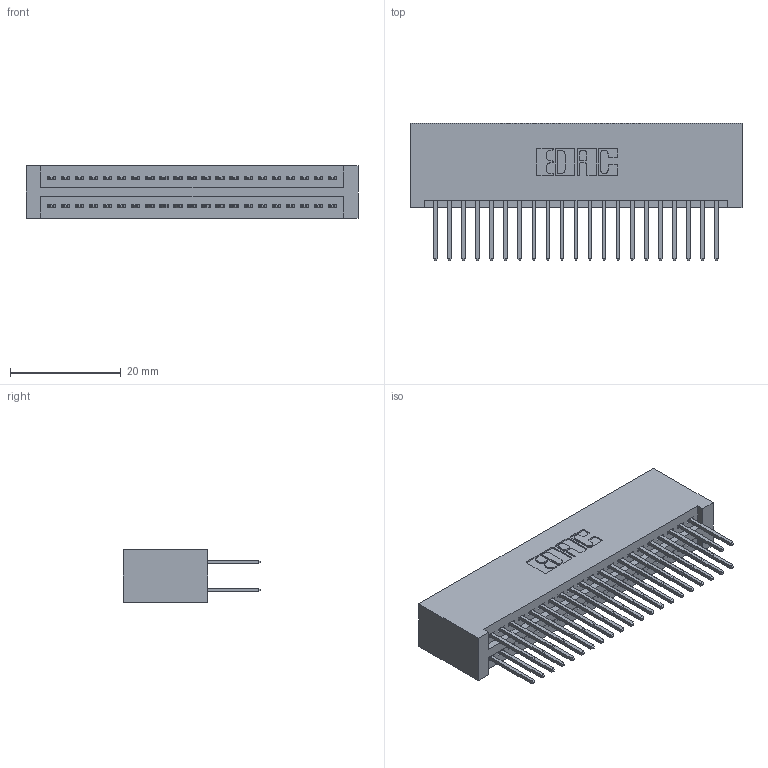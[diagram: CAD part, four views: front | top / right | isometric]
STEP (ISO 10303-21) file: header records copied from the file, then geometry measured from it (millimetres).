
FILE_DESCRIPTION (( 'STEP AP203' ), '1' );
FILE_NAME ('395-042-523-201.STEP', '2019-10-18T06:40:13', ( '' ), ( '' ), 'SwSTEP 2.0', 'SolidWorks 2016', '' );
FILE_SCHEMA (( 'CONFIG_CONTROL_DESIGN' ));
Length unit declared in the file: inch
Products named in the file (3): 395-042-523-201; 345 Part_No Mounting Lugs; 345-292-001_345-293-123
Assembly tree (43 placements, depth 2):
  395-042-523-201
    345 Part_No Mounting Lugs
    345-292-001_345-293-123  x42
Bounding box: 59.94 x 24.82 x 9.4 mm (x, y, z)
Volume: 6330.1 mm3; surface area: 9639.6 mm2
Topology: 43 solids, 43 shells, 2218 faces, 6575 edges, 4326 vertices
Faces by surface type: plane 1462, cylinder 756
Entity records: 19045 total; most frequent: CARTESIAN_POINT 3212, ORIENTED_EDGE 3146, DIRECTION 2853, EDGE_CURVE 1573, VECTOR 1365, LINE 1365, VERTEX_POINT 1046, AXIS2_PLACEMENT_3D 744
